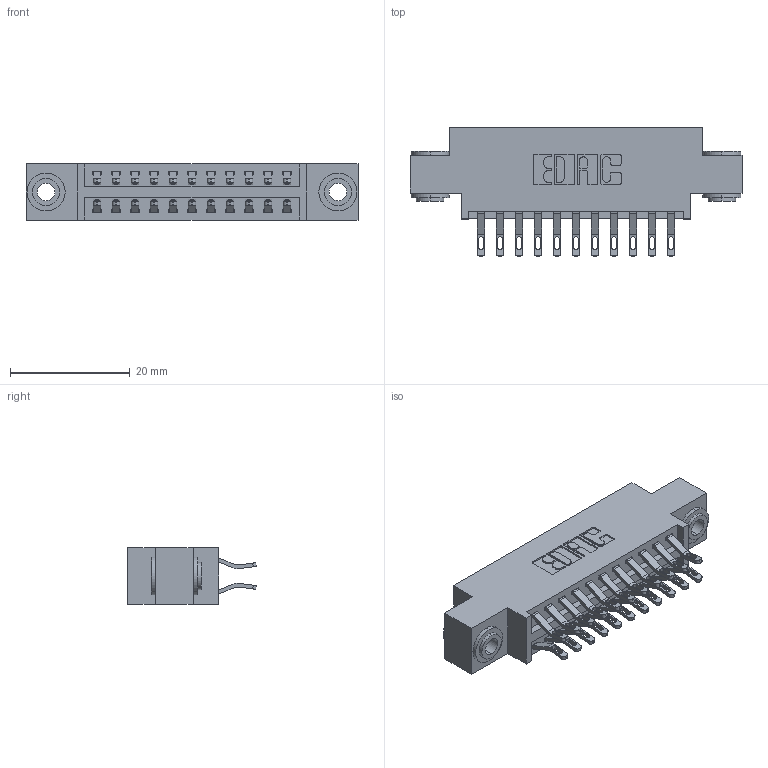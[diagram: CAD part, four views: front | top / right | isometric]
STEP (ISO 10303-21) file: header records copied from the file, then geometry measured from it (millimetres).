
FILE_DESCRIPTION (( 'STEP AP203' ), '1' );
FILE_NAME ('346-022-555-803.STEP', '2022-05-18T21:42:50', ( '' ), ( '' ), 'SwSTEP 2.0', 'SolidWorks 2020', '' );
FILE_SCHEMA (( 'CONFIG_CONTROL_DESIGN' ));
Length unit declared in the file: inch
Products named in the file (4): 345-250-002_345-250-002-102; 345-292-001_555 Tail; 346-022-555-803; 346 Part_0.170 Offset - 0.156 Dia-TH
Assembly tree (25 placements, depth 2):
  346-022-555-803
    346 Part_0.170 Offset - 0.156 Dia-TH
    345-292-001_555 Tail  x22
    345-250-002_345-250-002-102  x2
Bounding box: 55.5 x 21.46 x 9.4 mm (x, y, z)
Volume: 5081.6 mm3; surface area: 7153.5 mm2
Topology: 25 solids, 25 shells, 1454 faces, 4479 edges, 2982 vertices
Faces by surface type: plane 830, cylinder 616, cone 8
Entity records: 12876 total; most frequent: CARTESIAN_POINT 2183, ORIENTED_EDGE 2078, DIRECTION 1973, EDGE_CURVE 1039, VECTOR 819, LINE 819, VERTEX_POINT 690, AXIS2_PLACEMENT_3D 577
